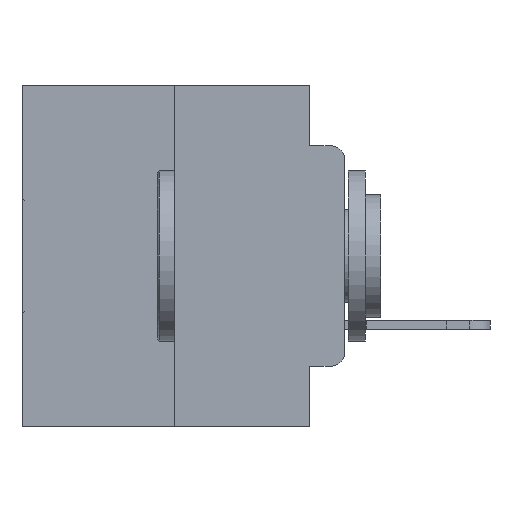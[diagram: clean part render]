
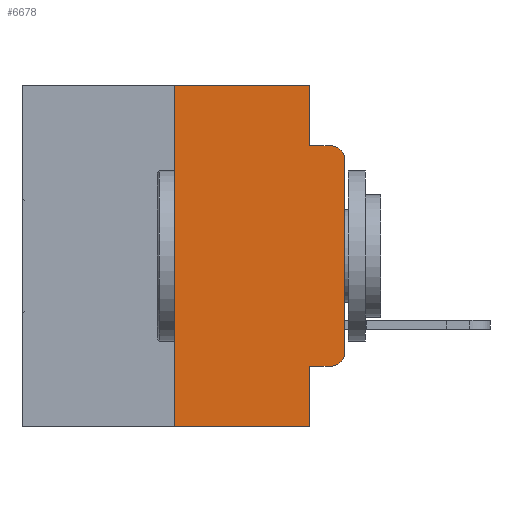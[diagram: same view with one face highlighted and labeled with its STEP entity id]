
A CAD part, left-side view. The second image highlights one B-rep face of the part: STEP entity #6678.
In plain terms, the highlighted planar face has unit normal (-1, 0, 0).
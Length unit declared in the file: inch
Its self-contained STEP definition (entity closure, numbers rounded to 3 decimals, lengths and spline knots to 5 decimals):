
#933 = CARTESIAN_POINT ( 'NONE',  ( 0., 0.051, -0.5 ) ) ;
#1612 = DIRECTION ( 'NONE',  ( 0., -1., 0. ) ) ;
#2025 = CARTESIAN_POINT ( 'NONE',  ( 0., 0.051, -0.4115 ) ) ;
#3258 = VERTEX_POINT ( 'NONE', #10044 ) ;
#4545 = EDGE_CURVE ( 'NONE', #27069, #21696, #5239, .T. ) ;
#4884 = ORIENTED_EDGE ( 'NONE', *, *, #7012, .T. ) ;
#5085 = ORIENTED_EDGE ( 'NONE', *, *, #7178, .F. ) ;
#5099 = LINE ( 'NONE', #15271, #30389 ) ;
#5139 = DIRECTION ( 'NONE',  ( 0., -1., 0. ) ) ;
#5239 = LINE ( 'NONE', #28206, #29856 ) ;
#5315 = EDGE_LOOP ( 'NONE', ( #4884, #5672, #15095, #5085, #20245, #5332, #8388, #20783, #18105, #15248 ) ) ;
#5332 = ORIENTED_EDGE ( 'NONE', *, *, #7232, .F. ) ;
#5672 = ORIENTED_EDGE ( 'NONE', *, *, #7068, .T. ) ;
#5687 = CARTESIAN_POINT ( 'NONE',  ( 0., 0.473, 0. ) ) ;
#5849 = CARTESIAN_POINT ( 'NONE',  ( 0., 0.25, 0. ) ) ;
#5917 = CARTESIAN_POINT ( 'NONE',  ( 0., 0.25, 0. ) ) ;
#6093 = DIRECTION ( 'NONE',  ( 0., 0., 1. ) ) ;
#6678 = ADVANCED_FACE ( 'NONE', ( #8918 ), #31262, .F. ) ;
#7012 = EDGE_CURVE ( 'NONE', #30531, #22805, #26498, .T. ) ;
#7068 = EDGE_CURVE ( 'NONE', #22805, #23144, #12449, .T. ) ;
#7113 = EDGE_CURVE ( 'NONE', #28265, #23144, #23763, .T. ) ;
#7178 = EDGE_CURVE ( 'NONE', #3258, #28265, #14428, .T. ) ;
#7232 = EDGE_CURVE ( 'NONE', #27069, #15778, #12829, .T. ) ;
#7282 = DIRECTION ( 'NONE',  ( 0., 0., -1. ) ) ;
#7357 = CARTESIAN_POINT ( 'NONE',  ( 0., 0.051, 0. ) ) ;
#7673 = EDGE_CURVE ( 'NONE', #21088, #21696, #5099, .T. ) ;
#7870 = EDGE_CURVE ( 'NONE', #21088, #10992, #10807, .T. ) ;
#8027 = EDGE_CURVE ( 'NONE', #10992, #30531, #17795, .T. ) ;
#8388 = ORIENTED_EDGE ( 'NONE', *, *, #4545, .T. ) ;
#8815 = CARTESIAN_POINT ( 'NONE',  ( 0., 0., -0.1085 ) ) ;
#8918 = FACE_OUTER_BOUND ( 'NONE', #5315, .T. ) ;
#9483 = EDGE_CURVE ( 'NONE', #15778, #3258, #30620, .T. ) ;
#9881 = CARTESIAN_POINT ( 'NONE',  ( 0., 0.25, -0.5 ) ) ;
#10044 = CARTESIAN_POINT ( 'NONE',  ( 0., 0.051, 0. ) ) ;
#10183 = DIRECTION ( 'NONE',  ( 0., -1., 0. ) ) ;
#10252 = CARTESIAN_POINT ( 'NONE',  ( 0., 0.051, -0.0885 ) ) ;
#10807 = LINE ( 'NONE', #2025, #28782 ) ;
#10843 = DIRECTION ( 'NONE',  ( 0., 0., -1. ) ) ;
#10870 = VECTOR ( 'NONE', #10183, 39.37008 ) ;
#10887 = DIRECTION ( 'NONE',  ( -1., 0., 0. ) ) ;
#10934 = AXIS2_PLACEMENT_3D ( 'NONE', #31169, #31145, #31123 ) ;
#10959 = CARTESIAN_POINT ( 'NONE',  ( 0., 0.02, -0.1085 ) ) ;
#10992 = VERTEX_POINT ( 'NONE', #11051 ) ;
#11051 = CARTESIAN_POINT ( 'NONE',  ( 0., 0.02, -0.4115 ) ) ;
#12041 = VECTOR ( 'NONE', #6093, 39.37008 ) ;
#12449 = CIRCLE ( 'NONE', #16373, 0.02 ) ;
#12829 = LINE ( 'NONE', #5917, #12041 ) ;
#13125 = DIRECTION ( 'NONE',  ( 0., 0., 1. ) ) ;
#13231 = CARTESIAN_POINT ( 'NONE',  ( 0., 0., 0. ) ) ;
#14049 = VECTOR ( 'NONE', #13125, 39.37008 ) ;
#14150 = CARTESIAN_POINT ( 'NONE',  ( 0., 0.051, -0.4115 ) ) ;
#14428 = LINE ( 'NONE', #7357, #26144 ) ;
#15028 = DIRECTION ( 'NONE',  ( 0., 0., -1. ) ) ;
#15095 = ORIENTED_EDGE ( 'NONE', *, *, #7113, .F. ) ;
#15248 = ORIENTED_EDGE ( 'NONE', *, *, #8027, .T. ) ;
#15271 = CARTESIAN_POINT ( 'NONE',  ( 0., 0.051, 0. ) ) ;
#15618 = AXIS2_PLACEMENT_3D ( 'NONE', #28350, #28345, #28253 ) ;
#15778 = VERTEX_POINT ( 'NONE', #5849 ) ;
#16373 = AXIS2_PLACEMENT_3D ( 'NONE', #10959, #10887, #10843 ) ;
#17795 = CIRCLE ( 'NONE', #15618, 0.02 ) ;
#18105 = ORIENTED_EDGE ( 'NONE', *, *, #7870, .T. ) ;
#20245 = ORIENTED_EDGE ( 'NONE', *, *, #9483, .F. ) ;
#20783 = ORIENTED_EDGE ( 'NONE', *, *, #7673, .F. ) ;
#21088 = VERTEX_POINT ( 'NONE', #14150 ) ;
#21696 = VERTEX_POINT ( 'NONE', #933 ) ;
#22805 = VERTEX_POINT ( 'NONE', #8815 ) ;
#23144 = VERTEX_POINT ( 'NONE', #30724 ) ;
#23763 = LINE ( 'NONE', #10252, #10870 ) ;
#25000 = VECTOR ( 'NONE', #5139, 39.37008 ) ;
#25931 = CARTESIAN_POINT ( 'NONE',  ( 0., 0., -0.3915 ) ) ;
#26144 = VECTOR ( 'NONE', #7282, 39.37008 ) ;
#26498 = LINE ( 'NONE', #13231, #14049 ) ;
#27069 = VERTEX_POINT ( 'NONE', #9881 ) ;
#27845 = DIRECTION ( 'NONE',  ( 0., -1., 0. ) ) ;
#27915 = CARTESIAN_POINT ( 'NONE',  ( 0., 0.051, -0.0885 ) ) ;
#28206 = CARTESIAN_POINT ( 'NONE',  ( 0., 0.473, -0.5 ) ) ;
#28253 = DIRECTION ( 'NONE',  ( 0., 0., -1. ) ) ;
#28265 = VERTEX_POINT ( 'NONE', #27915 ) ;
#28345 = DIRECTION ( 'NONE',  ( -1., 0., 0. ) ) ;
#28350 = CARTESIAN_POINT ( 'NONE',  ( 0., 0.02, -0.3915 ) ) ;
#28782 = VECTOR ( 'NONE', #1612, 39.37008 ) ;
#29856 = VECTOR ( 'NONE', #27845, 39.37008 ) ;
#30389 = VECTOR ( 'NONE', #15028, 39.37008 ) ;
#30531 = VERTEX_POINT ( 'NONE', #25931 ) ;
#30620 = LINE ( 'NONE', #5687, #25000 ) ;
#30724 = CARTESIAN_POINT ( 'NONE',  ( 0., 0.02, -0.0885 ) ) ;
#31123 = DIRECTION ( 'NONE',  ( 0., 0., -1. ) ) ;
#31145 = DIRECTION ( 'NONE',  ( 1., 0., 0. ) ) ;
#31169 = CARTESIAN_POINT ( 'NONE',  ( 0., 0.473, 0. ) ) ;
#31262 = PLANE ( 'NONE',  #10934 ) ;
